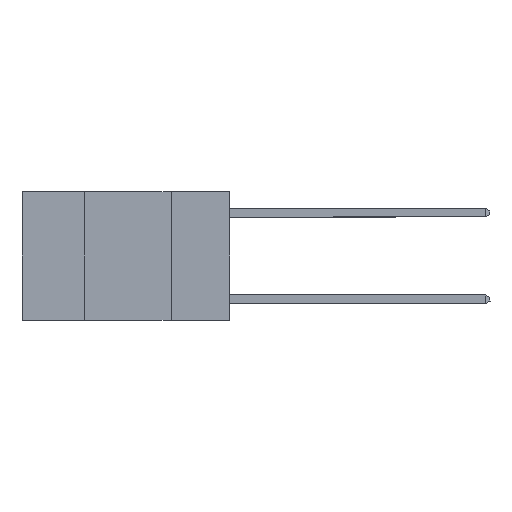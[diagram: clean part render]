
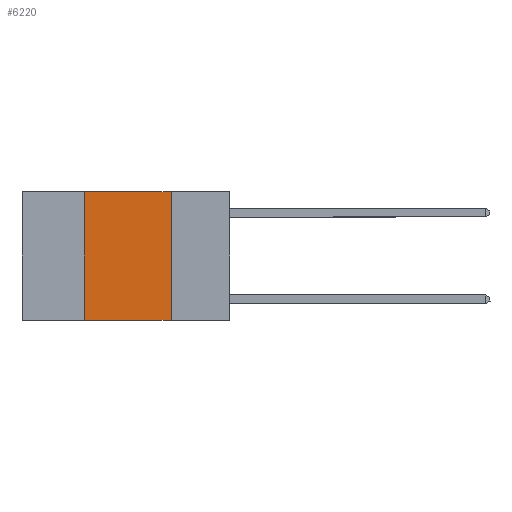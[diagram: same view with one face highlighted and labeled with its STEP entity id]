
A CAD part, left-side view. The second image highlights one B-rep face of the part: STEP entity #6220.
In plain terms, the highlighted planar face has unit normal (-1, 0, 0).
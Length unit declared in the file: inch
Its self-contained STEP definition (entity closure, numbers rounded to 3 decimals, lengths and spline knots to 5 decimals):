
#59 = EDGE_CURVE ( 'NONE', #11014, #8032, #2567, .T. ) ;
#879 = VECTOR ( 'NONE', #9032, 39.37008 ) ;
#978 = CARTESIAN_POINT ( 'NONE',  ( 0., 0.6, 0. ) ) ;
#1544 = VERTEX_POINT ( 'NONE', #6277 ) ;
#2275 = VECTOR ( 'NONE', #9315, 39.37008 ) ;
#2435 = EDGE_CURVE ( 'NONE', #9768, #1544, #7006, .T. ) ;
#2567 = LINE ( 'NONE', #8938, #2275 ) ;
#3063 = EDGE_LOOP ( 'NONE', ( #10663, #10852, #8715, #9471 ) ) ;
#3801 = CARTESIAN_POINT ( 'NONE',  ( 0., 0.17, 0. ) ) ;
#3869 = DIRECTION ( 'NONE',  ( 0., 0., -1. ) ) ;
#5575 = LINE ( 'NONE', #8217, #879 ) ;
#6220 = ADVANCED_FACE ( 'NONE', ( #10742 ), #7404, .F. ) ;
#6277 = CARTESIAN_POINT ( 'NONE',  ( 0., 0.42, 0. ) ) ;
#6760 = CARTESIAN_POINT ( 'NONE',  ( 0., 0.17, -0.37 ) ) ;
#6848 = EDGE_CURVE ( 'NONE', #1544, #11014, #8007, .T. ) ;
#7006 = LINE ( 'NONE', #9596, #9223 ) ;
#7210 = DIRECTION ( 'NONE',  ( 0., -1., 0. ) ) ;
#7404 = PLANE ( 'NONE',  #9260 ) ;
#8007 = LINE ( 'NONE', #978, #10208 ) ;
#8032 = VERTEX_POINT ( 'NONE', #6760 ) ;
#8217 = CARTESIAN_POINT ( 'NONE',  ( 0., 0.6, -0.37 ) ) ;
#8623 = CARTESIAN_POINT ( 'NONE',  ( 0., 0.42, -0.37 ) ) ;
#8715 = ORIENTED_EDGE ( 'NONE', *, *, #2435, .F. ) ;
#8938 = CARTESIAN_POINT ( 'NONE',  ( 0., 0.17, 0. ) ) ;
#9032 = DIRECTION ( 'NONE',  ( 0., -1., 0. ) ) ;
#9081 = DIRECTION ( 'NONE',  ( 1., 0., 0. ) ) ;
#9223 = VECTOR ( 'NONE', #10430, 39.37008 ) ;
#9260 = AXIS2_PLACEMENT_3D ( 'NONE', #10727, #9081, #3869 ) ;
#9315 = DIRECTION ( 'NONE',  ( 0., 0., -1. ) ) ;
#9471 = ORIENTED_EDGE ( 'NONE', *, *, #10160, .T. ) ;
#9596 = CARTESIAN_POINT ( 'NONE',  ( 0., 0.42, 0. ) ) ;
#9768 = VERTEX_POINT ( 'NONE', #8623 ) ;
#10160 = EDGE_CURVE ( 'NONE', #9768, #8032, #5575, .T. ) ;
#10208 = VECTOR ( 'NONE', #7210, 39.37008 ) ;
#10430 = DIRECTION ( 'NONE',  ( 0., 0., 1. ) ) ;
#10663 = ORIENTED_EDGE ( 'NONE', *, *, #59, .F. ) ;
#10727 = CARTESIAN_POINT ( 'NONE',  ( 0., 0.6, 0. ) ) ;
#10742 = FACE_OUTER_BOUND ( 'NONE', #3063, .T. ) ;
#10852 = ORIENTED_EDGE ( 'NONE', *, *, #6848, .F. ) ;
#11014 = VERTEX_POINT ( 'NONE', #3801 ) ;
